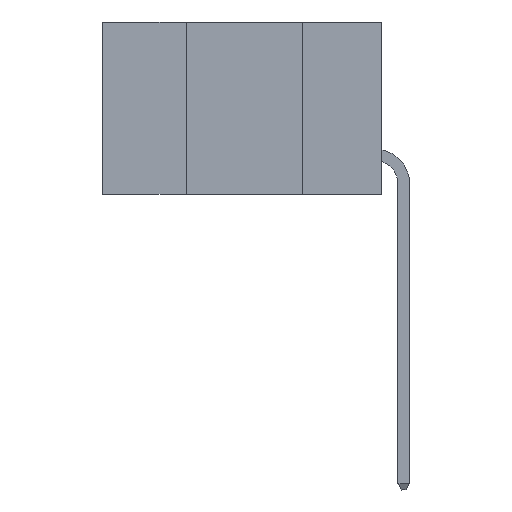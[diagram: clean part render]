
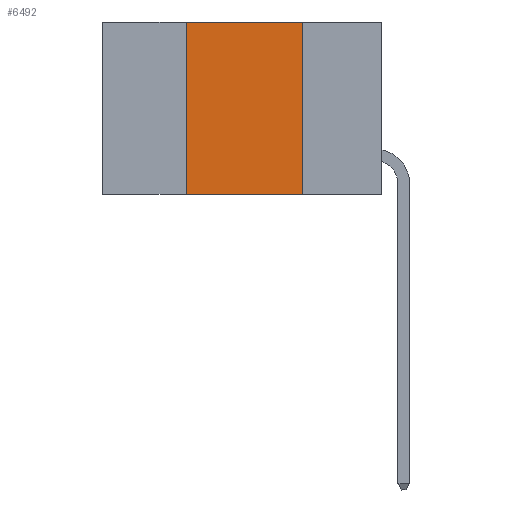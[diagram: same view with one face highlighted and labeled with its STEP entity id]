
A CAD part, left-side view. The second image highlights one B-rep face of the part: STEP entity #6492.
In plain terms, the highlighted planar face has unit normal (-1, 0, 0).
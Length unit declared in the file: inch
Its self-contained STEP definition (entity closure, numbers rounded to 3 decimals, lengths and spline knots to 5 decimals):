
#79 = VERTEX_POINT ( 'NONE', #1149 ) ;
#247 = VECTOR ( 'NONE', #11264, 39.37008 ) ;
#308 = FACE_OUTER_BOUND ( 'NONE', #5634, .T. ) ;
#1149 = CARTESIAN_POINT ( 'NONE',  ( 0., 0.17, -0.37 ) ) ;
#1966 = DIRECTION ( 'NONE',  ( 0., -1., 0. ) ) ;
#2088 = AXIS2_PLACEMENT_3D ( 'NONE', #8876, #10798, #5088 ) ;
#2714 = CARTESIAN_POINT ( 'NONE',  ( 0., 0.42, 0. ) ) ;
#2924 = CARTESIAN_POINT ( 'NONE',  ( 0., 0.6, 0. ) ) ;
#3658 = ORIENTED_EDGE ( 'NONE', *, *, #8826, .F. ) ;
#3943 = ORIENTED_EDGE ( 'NONE', *, *, #5042, .F. ) ;
#4128 = PLANE ( 'NONE',  #2088 ) ;
#4547 = DIRECTION ( 'NONE',  ( 0., 0., 1. ) ) ;
#4703 = VECTOR ( 'NONE', #4547, 39.37008 ) ;
#5042 = EDGE_CURVE ( 'NONE', #6189, #7751, #9708, .T. ) ;
#5088 = DIRECTION ( 'NONE',  ( 0., 0., -1. ) ) ;
#5634 = EDGE_LOOP ( 'NONE', ( #3658, #3943, #9039, #11572 ) ) ;
#5804 = CARTESIAN_POINT ( 'NONE',  ( 0., 0.42, -0.37 ) ) ;
#5880 = LINE ( 'NONE', #10322, #247 ) ;
#6189 = VERTEX_POINT ( 'NONE', #2714 ) ;
#6442 = CARTESIAN_POINT ( 'NONE',  ( 0., 0.42, 0. ) ) ;
#6492 = ADVANCED_FACE ( 'NONE', ( #308 ), #4128, .F. ) ;
#6929 = EDGE_CURVE ( 'NONE', #9525, #6189, #7244, .T. ) ;
#7244 = LINE ( 'NONE', #6442, #4703 ) ;
#7352 = VECTOR ( 'NONE', #1966, 39.37008 ) ;
#7687 = CARTESIAN_POINT ( 'NONE',  ( 0., 0.17, 0. ) ) ;
#7751 = VERTEX_POINT ( 'NONE', #7687 ) ;
#8429 = EDGE_CURVE ( 'NONE', #9525, #79, #12411, .T. ) ;
#8655 = DIRECTION ( 'NONE',  ( 0., -1., 0. ) ) ;
#8826 = EDGE_CURVE ( 'NONE', #7751, #79, #5880, .T. ) ;
#8876 = CARTESIAN_POINT ( 'NONE',  ( 0., 0.6, 0. ) ) ;
#9039 = ORIENTED_EDGE ( 'NONE', *, *, #6929, .F. ) ;
#9525 = VERTEX_POINT ( 'NONE', #5804 ) ;
#9708 = LINE ( 'NONE', #2924, #12228 ) ;
#9710 = CARTESIAN_POINT ( 'NONE',  ( 0., 0.6, -0.37 ) ) ;
#10322 = CARTESIAN_POINT ( 'NONE',  ( 0., 0.17, 0. ) ) ;
#10798 = DIRECTION ( 'NONE',  ( 1., 0., 0. ) ) ;
#11264 = DIRECTION ( 'NONE',  ( 0., 0., -1. ) ) ;
#11572 = ORIENTED_EDGE ( 'NONE', *, *, #8429, .T. ) ;
#12228 = VECTOR ( 'NONE', #8655, 39.37008 ) ;
#12411 = LINE ( 'NONE', #9710, #7352 ) ;
